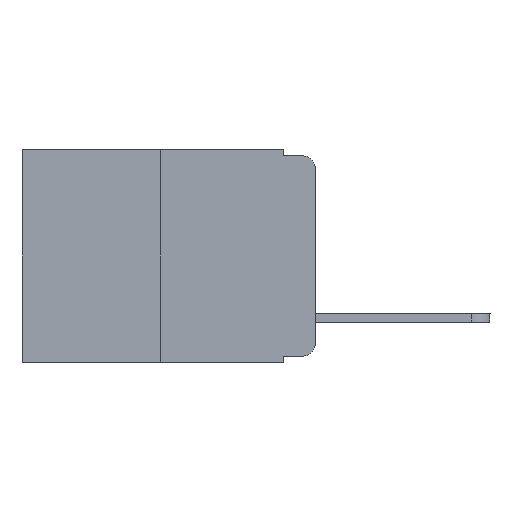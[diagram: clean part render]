
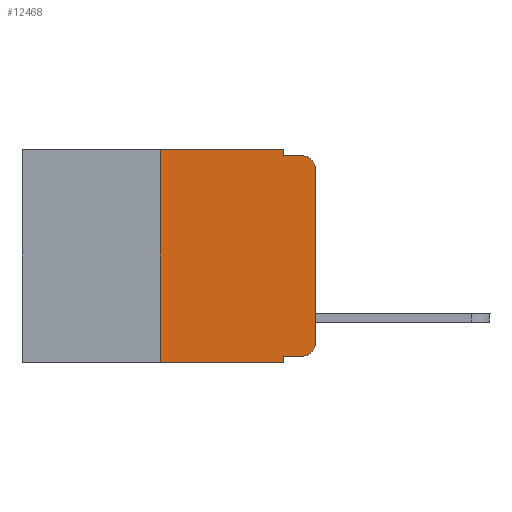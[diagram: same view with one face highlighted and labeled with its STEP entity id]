
A CAD part, left-side view. The second image highlights one B-rep face of the part: STEP entity #12468.
In plain terms, the highlighted planar face has unit normal (-1, 0, 0).
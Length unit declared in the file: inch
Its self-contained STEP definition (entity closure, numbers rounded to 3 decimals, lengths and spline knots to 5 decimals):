
#369 = CARTESIAN_POINT ( 'NONE',  ( 0., 0.051, -0.333 ) ) ;
#820 = VERTEX_POINT ( 'NONE', #21442 ) ;
#1482 = VECTOR ( 'NONE', #10178, 39.37008 ) ;
#1679 = CARTESIAN_POINT ( 'NONE',  ( 0., 0.02, -0.333 ) ) ;
#1891 = ORIENTED_EDGE ( 'NONE', *, *, #5036, .F. ) ;
#1921 = ORIENTED_EDGE ( 'NONE', *, *, #3521, .F. ) ;
#2130 = VERTEX_POINT ( 'NONE', #23425 ) ;
#2457 = PLANE ( 'NONE',  #18515 ) ;
#2583 = FACE_OUTER_BOUND ( 'NONE', #12678, .T. ) ;
#2639 = CARTESIAN_POINT ( 'NONE',  ( 0., 0.051, 0. ) ) ;
#2986 = ORIENTED_EDGE ( 'NONE', *, *, #6563, .T. ) ;
#3064 = EDGE_CURVE ( 'NONE', #11186, #10579, #22302, .T. ) ;
#3379 = LINE ( 'NONE', #5073, #13270 ) ;
#3493 = DIRECTION ( 'NONE',  ( 0., 0., 1. ) ) ;
#3521 = EDGE_CURVE ( 'NONE', #2130, #5632, #23499, .T. ) ;
#3874 = VERTEX_POINT ( 'NONE', #22218 ) ;
#3932 = CARTESIAN_POINT ( 'NONE',  ( 0., 0.473, -0.343 ) ) ;
#3955 = VECTOR ( 'NONE', #19888, 39.37008 ) ;
#4270 = DIRECTION ( 'NONE',  ( 1., 0., 0. ) ) ;
#4329 = CARTESIAN_POINT ( 'NONE',  ( 0., 0.02, -0.01 ) ) ;
#4494 = DIRECTION ( 'NONE',  ( 0., 0., -1. ) ) ;
#5036 = EDGE_CURVE ( 'NONE', #12400, #11661, #11885, .T. ) ;
#5073 = CARTESIAN_POINT ( 'NONE',  ( 0., 0.051, -0.333 ) ) ;
#5632 = VERTEX_POINT ( 'NONE', #10623 ) ;
#5713 = CARTESIAN_POINT ( 'NONE',  ( 0., 0.051, 0. ) ) ;
#5901 = VECTOR ( 'NONE', #14294, 39.37008 ) ;
#6175 = DIRECTION ( 'NONE',  ( -1., 0., 0. ) ) ;
#6553 = VERTEX_POINT ( 'NONE', #19247 ) ;
#6563 = EDGE_CURVE ( 'NONE', #10360, #3874, #6907, .T. ) ;
#6899 = CARTESIAN_POINT ( 'NONE',  ( 0., 0.473, 0. ) ) ;
#6907 = CIRCLE ( 'NONE', #21590, 0.02 ) ;
#7116 = EDGE_CURVE ( 'NONE', #3874, #6553, #21261, .T. ) ;
#7243 = ORIENTED_EDGE ( 'NONE', *, *, #3064, .F. ) ;
#7573 = LINE ( 'NONE', #3932, #20384 ) ;
#8599 = CARTESIAN_POINT ( 'NONE',  ( 0., 0.051, -0.01 ) ) ;
#8934 = EDGE_CURVE ( 'NONE', #6553, #11661, #19410, .T. ) ;
#9028 = DIRECTION ( 'NONE',  ( 0., 0., -1. ) ) ;
#9264 = DIRECTION ( 'NONE',  ( -1., 0., 0. ) ) ;
#10021 = DIRECTION ( 'NONE',  ( 0., 0., -1. ) ) ;
#10178 = DIRECTION ( 'NONE',  ( 0., -1., 0. ) ) ;
#10277 = EDGE_CURVE ( 'NONE', #820, #10579, #7573, .T. ) ;
#10360 = VERTEX_POINT ( 'NONE', #1679 ) ;
#10579 = VERTEX_POINT ( 'NONE', #18113 ) ;
#10623 = CARTESIAN_POINT ( 'NONE',  ( 0., 0.051, 0. ) ) ;
#11186 = VERTEX_POINT ( 'NONE', #369 ) ;
#11429 = EDGE_CURVE ( 'NONE', #820, #2130, #12706, .T. ) ;
#11661 = VERTEX_POINT ( 'NONE', #4329 ) ;
#11673 = DIRECTION ( 'NONE',  ( 0., 0., -1. ) ) ;
#11885 = LINE ( 'NONE', #8599, #1482 ) ;
#12400 = VERTEX_POINT ( 'NONE', #14931 ) ;
#12468 = ADVANCED_FACE ( 'NONE', ( #2583 ), #2457, .F. ) ;
#12501 = VECTOR ( 'NONE', #10021, 39.37008 ) ;
#12538 = ORIENTED_EDGE ( 'NONE', *, *, #15558, .T. ) ;
#12678 = EDGE_LOOP ( 'NONE', ( #22870, #14608, #1891, #22311, #1921, #13376, #20055, #7243, #12538, #2986 ) ) ;
#12706 = LINE ( 'NONE', #20061, #18160 ) ;
#13270 = VECTOR ( 'NONE', #17917, 39.37008 ) ;
#13376 = ORIENTED_EDGE ( 'NONE', *, *, #11429, .F. ) ;
#13778 = VECTOR ( 'NONE', #17539, 39.37008 ) ;
#14016 = AXIS2_PLACEMENT_3D ( 'NONE', #21955, #9264, #9028 ) ;
#14294 = DIRECTION ( 'NONE',  ( 0., -1., 0. ) ) ;
#14608 = ORIENTED_EDGE ( 'NONE', *, *, #8934, .T. ) ;
#14931 = CARTESIAN_POINT ( 'NONE',  ( 0., 0.051, -0.01 ) ) ;
#15558 = EDGE_CURVE ( 'NONE', #11186, #10360, #3379, .T. ) ;
#15951 = EDGE_CURVE ( 'NONE', #5632, #12400, #19213, .T. ) ;
#16954 = CARTESIAN_POINT ( 'NONE',  ( 0., 0.02, -0.313 ) ) ;
#17539 = DIRECTION ( 'NONE',  ( 0., 0., 1. ) ) ;
#17917 = DIRECTION ( 'NONE',  ( 0., -1., 0. ) ) ;
#18113 = CARTESIAN_POINT ( 'NONE',  ( 0., 0.051, -0.343 ) ) ;
#18160 = VECTOR ( 'NONE', #3493, 39.37008 ) ;
#18515 = AXIS2_PLACEMENT_3D ( 'NONE', #19158, #4270, #11673 ) ;
#19158 = CARTESIAN_POINT ( 'NONE',  ( 0., 0.473, 0. ) ) ;
#19213 = LINE ( 'NONE', #2639, #12501 ) ;
#19247 = CARTESIAN_POINT ( 'NONE',  ( 0., 0., -0.03 ) ) ;
#19410 = CIRCLE ( 'NONE', #14016, 0.02 ) ;
#19571 = CARTESIAN_POINT ( 'NONE',  ( 0., 0., 0. ) ) ;
#19888 = DIRECTION ( 'NONE',  ( 0., 0., -1. ) ) ;
#20055 = ORIENTED_EDGE ( 'NONE', *, *, #10277, .T. ) ;
#20061 = CARTESIAN_POINT ( 'NONE',  ( 0., 0.25, 0. ) ) ;
#20384 = VECTOR ( 'NONE', #22439, 39.37008 ) ;
#21261 = LINE ( 'NONE', #19571, #13778 ) ;
#21442 = CARTESIAN_POINT ( 'NONE',  ( 0., 0.25, -0.343 ) ) ;
#21590 = AXIS2_PLACEMENT_3D ( 'NONE', #16954, #6175, #4494 ) ;
#21955 = CARTESIAN_POINT ( 'NONE',  ( 0., 0.02, -0.03 ) ) ;
#22218 = CARTESIAN_POINT ( 'NONE',  ( 0., 0., -0.313 ) ) ;
#22302 = LINE ( 'NONE', #5713, #3955 ) ;
#22311 = ORIENTED_EDGE ( 'NONE', *, *, #15951, .F. ) ;
#22439 = DIRECTION ( 'NONE',  ( 0., -1., 0. ) ) ;
#22870 = ORIENTED_EDGE ( 'NONE', *, *, #7116, .T. ) ;
#23425 = CARTESIAN_POINT ( 'NONE',  ( 0., 0.25, 0. ) ) ;
#23499 = LINE ( 'NONE', #6899, #5901 ) ;
